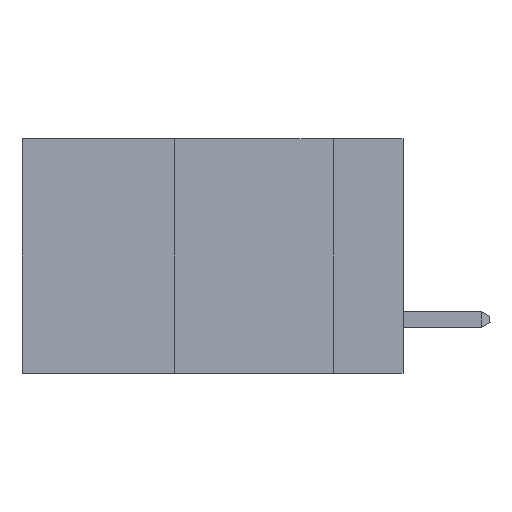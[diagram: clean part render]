
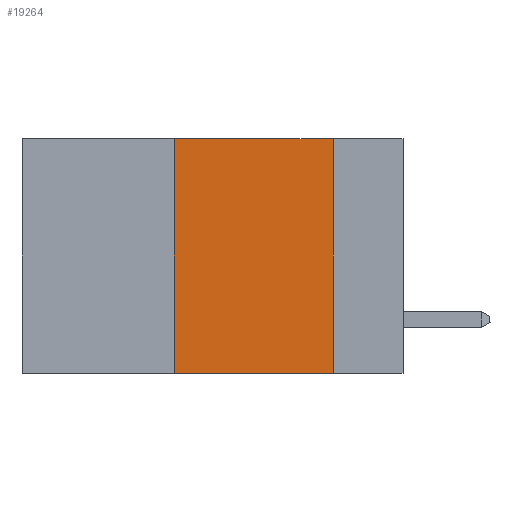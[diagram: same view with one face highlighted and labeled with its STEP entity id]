
A CAD part, left-side view. The second image highlights one B-rep face of the part: STEP entity #19264.
In plain terms, the highlighted planar face has unit normal (-1, 0, 0).
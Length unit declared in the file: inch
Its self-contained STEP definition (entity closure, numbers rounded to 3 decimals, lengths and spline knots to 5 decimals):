
#5 = VERTEX_POINT ( 'NONE', #5554 ) ;
#996 = ORIENTED_EDGE ( 'NONE', *, *, #19354, .F. ) ;
#1352 = CARTESIAN_POINT ( 'NONE',  ( 0., 0.36, 0. ) ) ;
#2045 = CARTESIAN_POINT ( 'NONE',  ( 0., 0.11, 0. ) ) ;
#2128 = DIRECTION ( 'NONE',  ( 1., 0., 0. ) ) ;
#2244 = ORIENTED_EDGE ( 'NONE', *, *, #8441, .T. ) ;
#2835 = LINE ( 'NONE', #3204, #12698 ) ;
#3204 = CARTESIAN_POINT ( 'NONE',  ( 0., 0.6, -0.37 ) ) ;
#4247 = ORIENTED_EDGE ( 'NONE', *, *, #17417, .F. ) ;
#4963 = DIRECTION ( 'NONE',  ( 0., -1., 0. ) ) ;
#5554 = CARTESIAN_POINT ( 'NONE',  ( 0., 0.36, 0. ) ) ;
#6074 = VECTOR ( 'NONE', #17902, 39.37008 ) ;
#6403 = LINE ( 'NONE', #2045, #6074 ) ;
#8064 = FACE_OUTER_BOUND ( 'NONE', #13970, .T. ) ;
#8441 = EDGE_CURVE ( 'NONE', #23690, #9616, #2835, .T. ) ;
#8800 = DIRECTION ( 'NONE',  ( 0., 0., 1. ) ) ;
#9616 = VERTEX_POINT ( 'NONE', #15760 ) ;
#9704 = DIRECTION ( 'NONE',  ( 0., 0., -1. ) ) ;
#10492 = VECTOR ( 'NONE', #18694, 39.37008 ) ;
#12574 = CARTESIAN_POINT ( 'NONE',  ( 0., 0.11, 0. ) ) ;
#12698 = VECTOR ( 'NONE', #4963, 39.37008 ) ;
#13485 = CARTESIAN_POINT ( 'NONE',  ( 0., 0.36, -0.37 ) ) ;
#13970 = EDGE_LOOP ( 'NONE', ( #4247, #996, #14271, #2244 ) ) ;
#14271 = ORIENTED_EDGE ( 'NONE', *, *, #21108, .F. ) ;
#15354 = VECTOR ( 'NONE', #8800, 39.37008 ) ;
#15760 = CARTESIAN_POINT ( 'NONE',  ( 0., 0.11, -0.37 ) ) ;
#17417 = EDGE_CURVE ( 'NONE', #23497, #9616, #6403, .T. ) ;
#17619 = LINE ( 'NONE', #24446, #10492 ) ;
#17902 = DIRECTION ( 'NONE',  ( 0., 0., -1. ) ) ;
#17968 = AXIS2_PLACEMENT_3D ( 'NONE', #21497, #2128, #9704 ) ;
#18694 = DIRECTION ( 'NONE',  ( 0., -1., 0. ) ) ;
#19264 = ADVANCED_FACE ( 'NONE', ( #8064 ), #24976, .F. ) ;
#19354 = EDGE_CURVE ( 'NONE', #5, #23497, #17619, .T. ) ;
#21108 = EDGE_CURVE ( 'NONE', #23690, #5, #23699, .T. ) ;
#21497 = CARTESIAN_POINT ( 'NONE',  ( 0., 0.6, 0. ) ) ;
#23497 = VERTEX_POINT ( 'NONE', #12574 ) ;
#23690 = VERTEX_POINT ( 'NONE', #13485 ) ;
#23699 = LINE ( 'NONE', #1352, #15354 ) ;
#24446 = CARTESIAN_POINT ( 'NONE',  ( 0., 0.6, 0. ) ) ;
#24976 = PLANE ( 'NONE',  #17968 ) ;
